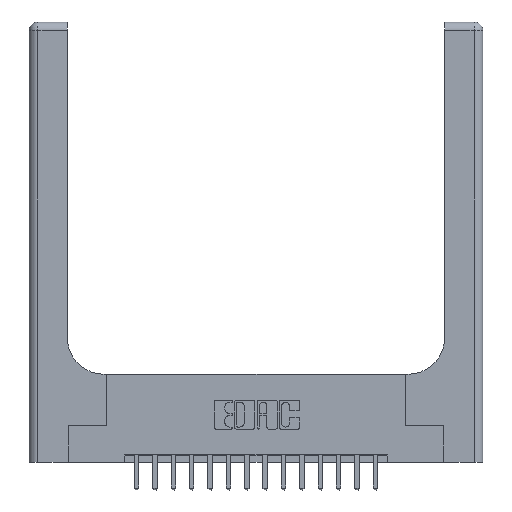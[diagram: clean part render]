
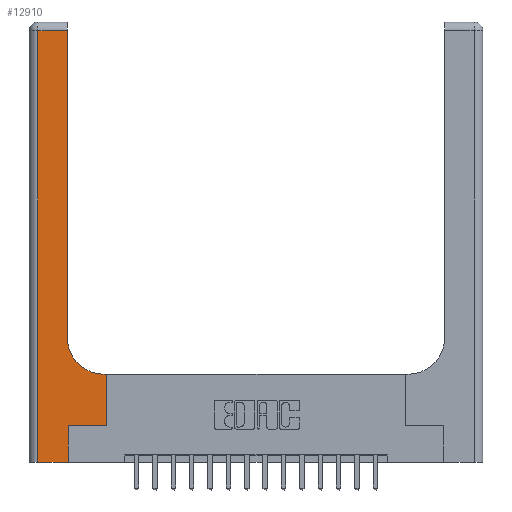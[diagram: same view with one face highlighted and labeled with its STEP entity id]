
A CAD part, top view. The second image highlights one B-rep face of the part: STEP entity #12910.
In plain terms, the highlighted planar face has unit normal (0, 0, 1).
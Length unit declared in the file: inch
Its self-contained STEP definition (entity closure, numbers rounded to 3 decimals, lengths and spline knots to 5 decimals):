
#27 = DIRECTION ( 'NONE',  ( -1., 0., 0. ) ) ;
#177 = DIRECTION ( 'NONE',  ( 0., 0., -1. ) ) ;
#179 = DIRECTION ( 'NONE',  ( -1., 0., 0. ) ) ;
#240 = VECTOR ( 'NONE', #16317, 39.37008 ) ;
#428 = ORIENTED_EDGE ( 'NONE', *, *, #8661, .T. ) ;
#434 = DIRECTION ( 'NONE',  ( 1., 0., 0. ) ) ;
#463 = VERTEX_POINT ( 'NONE', #5873 ) ;
#1223 = ORIENTED_EDGE ( 'NONE', *, *, #14084, .T. ) ;
#1461 = CARTESIAN_POINT ( 'NONE',  ( 0.265, 0., 0.37 ) ) ;
#1653 = CARTESIAN_POINT ( 'NONE',  ( 0.26, 3., 0.37 ) ) ;
#1849 = ORIENTED_EDGE ( 'NONE', *, *, #2334, .T. ) ;
#2334 = EDGE_CURVE ( 'NONE', #14933, #3088, #7260, .T. ) ;
#2712 = VECTOR ( 'NONE', #10306, 39.37008 ) ;
#2858 = CARTESIAN_POINT ( 'NONE',  ( 0.26, 2.94, 0.37 ) ) ;
#3088 = VERTEX_POINT ( 'NONE', #14650 ) ;
#3119 = CARTESIAN_POINT ( 'NONE',  ( 0.26, 0.6, 0.37 ) ) ;
#3842 = LINE ( 'NONE', #9597, #14703 ) ;
#3923 = DIRECTION ( 'NONE',  ( 0., -1., 0. ) ) ;
#4351 = ORIENTED_EDGE ( 'NONE', *, *, #8913, .T. ) ;
#4781 = VECTOR ( 'NONE', #27, 39.37008 ) ;
#4818 = EDGE_CURVE ( 'NONE', #12166, #5178, #6178, .T. ) ;
#4994 = CARTESIAN_POINT ( 'NONE',  ( 0.265, 0.25, 0.37 ) ) ;
#5178 = VERTEX_POINT ( 'NONE', #1461 ) ;
#5873 = CARTESIAN_POINT ( 'NONE',  ( 0.26, 0.85, 0.37 ) ) ;
#6080 = ORIENTED_EDGE ( 'NONE', *, *, #12211, .T. ) ;
#6178 = LINE ( 'NONE', #16245, #13298 ) ;
#7260 = LINE ( 'NONE', #14425, #4781 ) ;
#7295 = EDGE_CURVE ( 'NONE', #17372, #11075, #11888, .T. ) ;
#7652 = CARTESIAN_POINT ( 'NONE',  ( 0.265, 0.25, 0.37 ) ) ;
#8352 = VECTOR ( 'NONE', #179, 39.37008 ) ;
#8424 = VERTEX_POINT ( 'NONE', #13770 ) ;
#8661 = EDGE_CURVE ( 'NONE', #463, #14933, #10388, .T. ) ;
#8913 = EDGE_CURVE ( 'NONE', #8424, #463, #14143, .T. ) ;
#9083 = CARTESIAN_POINT ( 'NONE',  ( 0.06, 0., 0.37 ) ) ;
#9246 = CARTESIAN_POINT ( 'NONE',  ( 0.51, 0.85, 0.37 ) ) ;
#9252 = CARTESIAN_POINT ( 'NONE',  ( 0.528, 0.25, 0.37 ) ) ;
#9597 = CARTESIAN_POINT ( 'NONE',  ( 0.265, 0., 0.37 ) ) ;
#10076 = CARTESIAN_POINT ( 'NONE',  ( 0., 3., 0.37 ) ) ;
#10306 = DIRECTION ( 'NONE',  ( 0., 1., 0. ) ) ;
#10388 = LINE ( 'NONE', #1653, #2712 ) ;
#10578 = LINE ( 'NONE', #9252, #240 ) ;
#11075 = VERTEX_POINT ( 'NONE', #16610 ) ;
#11286 = FACE_OUTER_BOUND ( 'NONE', #12607, .T. ) ;
#11887 = CARTESIAN_POINT ( 'NONE',  ( 0.528, 0.6, 0.37 ) ) ;
#11888 = LINE ( 'NONE', #7652, #16724 ) ;
#12166 = VERTEX_POINT ( 'NONE', #9083 ) ;
#12211 = EDGE_CURVE ( 'NONE', #11075, #17055, #10578, .T. ) ;
#12328 = DIRECTION ( 'NONE',  ( 1., 0., 0. ) ) ;
#12607 = EDGE_LOOP ( 'NONE', ( #428, #1849, #14712, #14802, #13681, #18561, #6080, #1223, #4351 ) ) ;
#12910 = ADVANCED_FACE ( 'NONE', ( #11286 ), #14116, .F. ) ;
#13241 = AXIS2_PLACEMENT_3D ( 'NONE', #9246, #13461, #12328 ) ;
#13298 = VECTOR ( 'NONE', #434, 39.37008 ) ;
#13396 = DIRECTION ( 'NONE',  ( 1., 0., 0. ) ) ;
#13461 = DIRECTION ( 'NONE',  ( 0., 0., -1. ) ) ;
#13681 = ORIENTED_EDGE ( 'NONE', *, *, #14407, .T. ) ;
#13770 = CARTESIAN_POINT ( 'NONE',  ( 0.51, 0.6, 0.37 ) ) ;
#14084 = EDGE_CURVE ( 'NONE', #17055, #8424, #15623, .T. ) ;
#14116 = PLANE ( 'NONE',  #16824 ) ;
#14143 = CIRCLE ( 'NONE', #13241, 0.25 ) ;
#14407 = EDGE_CURVE ( 'NONE', #5178, #17372, #3842, .T. ) ;
#14425 = CARTESIAN_POINT ( 'NONE',  ( 0., 2.94, 0.37 ) ) ;
#14650 = CARTESIAN_POINT ( 'NONE',  ( 0.06, 2.94, 0.37 ) ) ;
#14703 = VECTOR ( 'NONE', #15219, 39.37008 ) ;
#14712 = ORIENTED_EDGE ( 'NONE', *, *, #15603, .T. ) ;
#14802 = ORIENTED_EDGE ( 'NONE', *, *, #4818, .T. ) ;
#14933 = VERTEX_POINT ( 'NONE', #2858 ) ;
#15219 = DIRECTION ( 'NONE',  ( 0., 1., 0. ) ) ;
#15496 = CARTESIAN_POINT ( 'NONE',  ( 0.06, 3., 0.37 ) ) ;
#15603 = EDGE_CURVE ( 'NONE', #3088, #12166, #16648, .T. ) ;
#15623 = LINE ( 'NONE', #3119, #8352 ) ;
#16171 = VECTOR ( 'NONE', #3923, 39.37008 ) ;
#16245 = CARTESIAN_POINT ( 'NONE',  ( 0., 0., 0.37 ) ) ;
#16317 = DIRECTION ( 'NONE',  ( 0., 1., 0. ) ) ;
#16610 = CARTESIAN_POINT ( 'NONE',  ( 0.528, 0.25, 0.37 ) ) ;
#16648 = LINE ( 'NONE', #15496, #16171 ) ;
#16724 = VECTOR ( 'NONE', #13396, 39.37008 ) ;
#16824 = AXIS2_PLACEMENT_3D ( 'NONE', #10076, #177, #16970 ) ;
#16970 = DIRECTION ( 'NONE',  ( -1., 0., 0. ) ) ;
#17055 = VERTEX_POINT ( 'NONE', #11887 ) ;
#17372 = VERTEX_POINT ( 'NONE', #4994 ) ;
#18561 = ORIENTED_EDGE ( 'NONE', *, *, #7295, .T. ) ;
